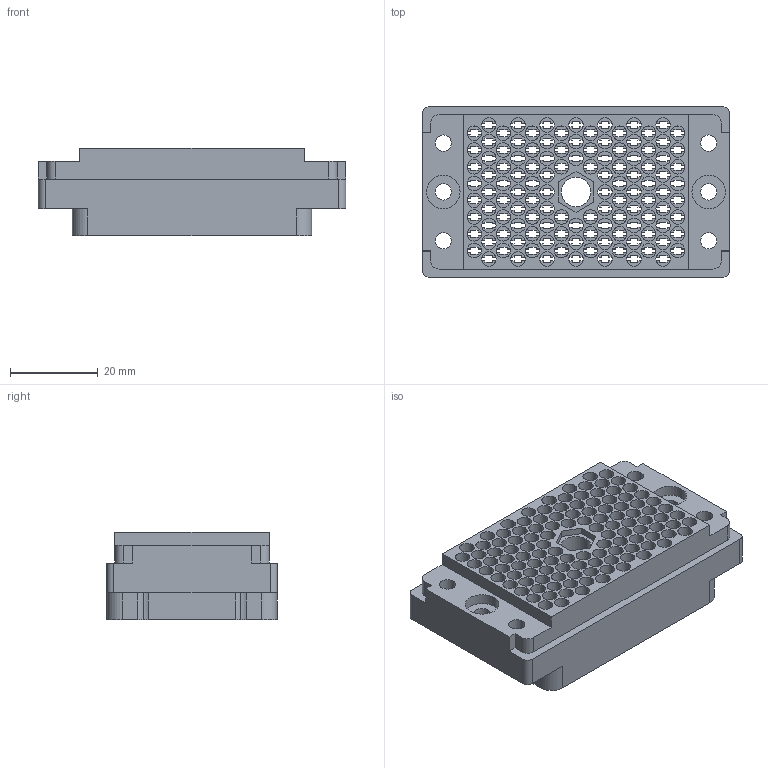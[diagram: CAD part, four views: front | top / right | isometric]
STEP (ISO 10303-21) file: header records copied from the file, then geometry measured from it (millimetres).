
FILE_DESCRIPTION (( 'STEP AP203' ), '1' );
FILE_NAME ('516-120-000-100.STEP', '2020-03-11T00:47:25', ( '' ), ( '' ), 'SwSTEP 2.0', 'SolidWorks 2016', '' );
FILE_SCHEMA (( 'CONFIG_CONTROL_DESIGN' ));
Length unit declared in the file: inch
Products named in the file (2): 516 Plug Insulator_120; 516-120-000-100
Assembly tree (1 placements, depth 2):
  516-120-000-100
    516 Plug Insulator_120
Bounding box: 69.85 x 38.73 x 19.81 mm (x, y, z)
Volume: 19275.8 mm3; surface area: 26896.6 mm2
Topology: 1 solids, 1 shells, 2378 faces, 7088 edges, 4724 vertices
Faces by surface type: plane 1799, cylinder 577, cone 2
Entity records: 80470 total; most frequent: CARTESIAN_POINT 14194, ORIENTED_EDGE 14176, DIRECTION 13494, EDGE_CURVE 7088, VECTOR 5446, LINE 5446, VERTEX_POINT 4724, AXIS2_PLACEMENT_3D 4024
